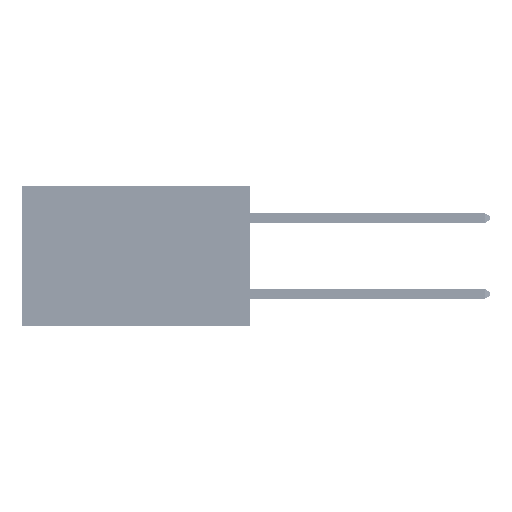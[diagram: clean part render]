
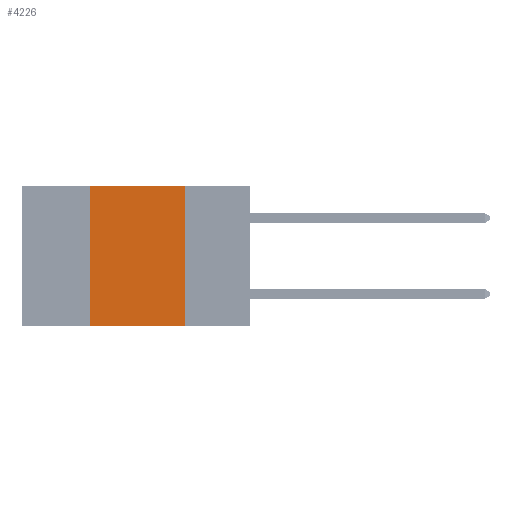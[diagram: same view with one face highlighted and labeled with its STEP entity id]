
A CAD part, left-side view. The second image highlights one B-rep face of the part: STEP entity #4226.
In plain terms, the highlighted planar face has unit normal (-1, 0, 0).
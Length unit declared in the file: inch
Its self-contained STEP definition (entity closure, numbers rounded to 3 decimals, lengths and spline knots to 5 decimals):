
#733 = DIRECTION ( 'NONE',  ( 0., 0., -1. ) ) ;
#966 = VECTOR ( 'NONE', #19778, 39.37008 ) ;
#2821 = FACE_OUTER_BOUND ( 'NONE', #23878, .T. ) ;
#3964 = ORIENTED_EDGE ( 'NONE', *, *, #21132, .F. ) ;
#4226 = ADVANCED_FACE ( 'NONE', ( #2821 ), #15230, .F. ) ;
#4605 = ORIENTED_EDGE ( 'NONE', *, *, #13958, .T. ) ;
#4850 = AXIS2_PLACEMENT_3D ( 'NONE', #40639, #40955, #7756 ) ;
#6109 = DIRECTION ( 'NONE',  ( 0., 0., 1. ) ) ;
#6792 = LINE ( 'NONE', #9528, #40388 ) ;
#7756 = DIRECTION ( 'NONE',  ( 0., 0., -1. ) ) ;
#8546 = CARTESIAN_POINT ( 'NONE',  ( 0., 0.6, 0. ) ) ;
#9528 = CARTESIAN_POINT ( 'NONE',  ( 0., 0.42, 0. ) ) ;
#13958 = EDGE_CURVE ( 'NONE', #35986, #28044, #22561, .T. ) ;
#13988 = ORIENTED_EDGE ( 'NONE', *, *, #29745, .F. ) ;
#15202 = EDGE_CURVE ( 'NONE', #34151, #24693, #35140, .T. ) ;
#15230 = PLANE ( 'NONE',  #4850 ) ;
#19778 = DIRECTION ( 'NONE',  ( 0., -1., 0. ) ) ;
#21132 = EDGE_CURVE ( 'NONE', #35986, #34151, #6792, .T. ) ;
#22561 = LINE ( 'NONE', #44921, #30056 ) ;
#23878 = EDGE_LOOP ( 'NONE', ( #13988, #35957, #3964, #4605 ) ) ;
#24693 = VERTEX_POINT ( 'NONE', #32738 ) ;
#27062 = VECTOR ( 'NONE', #733, 39.37008 ) ;
#28044 = VERTEX_POINT ( 'NONE', #39977 ) ;
#29745 = EDGE_CURVE ( 'NONE', #24693, #28044, #46759, .T. ) ;
#30056 = VECTOR ( 'NONE', #41839, 39.37008 ) ;
#30354 = CARTESIAN_POINT ( 'NONE',  ( 0., 0.17, 0. ) ) ;
#32738 = CARTESIAN_POINT ( 'NONE',  ( 0., 0.17, 0. ) ) ;
#34151 = VERTEX_POINT ( 'NONE', #44939 ) ;
#35140 = LINE ( 'NONE', #8546, #966 ) ;
#35957 = ORIENTED_EDGE ( 'NONE', *, *, #15202, .F. ) ;
#35986 = VERTEX_POINT ( 'NONE', #38078 ) ;
#38078 = CARTESIAN_POINT ( 'NONE',  ( 0., 0.42, -0.37 ) ) ;
#39977 = CARTESIAN_POINT ( 'NONE',  ( 0., 0.17, -0.37 ) ) ;
#40388 = VECTOR ( 'NONE', #6109, 39.37008 ) ;
#40639 = CARTESIAN_POINT ( 'NONE',  ( 0., 0.6, 0. ) ) ;
#40955 = DIRECTION ( 'NONE',  ( 1., 0., 0. ) ) ;
#41839 = DIRECTION ( 'NONE',  ( 0., -1., 0. ) ) ;
#44921 = CARTESIAN_POINT ( 'NONE',  ( 0., 0.6, -0.37 ) ) ;
#44939 = CARTESIAN_POINT ( 'NONE',  ( 0., 0.42, 0. ) ) ;
#46759 = LINE ( 'NONE', #30354, #27062 ) ;
